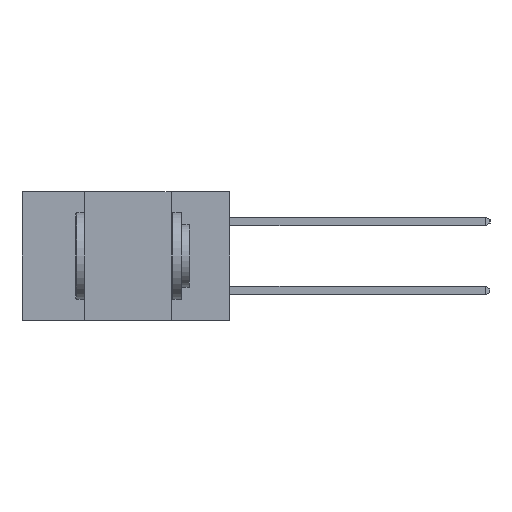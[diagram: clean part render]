
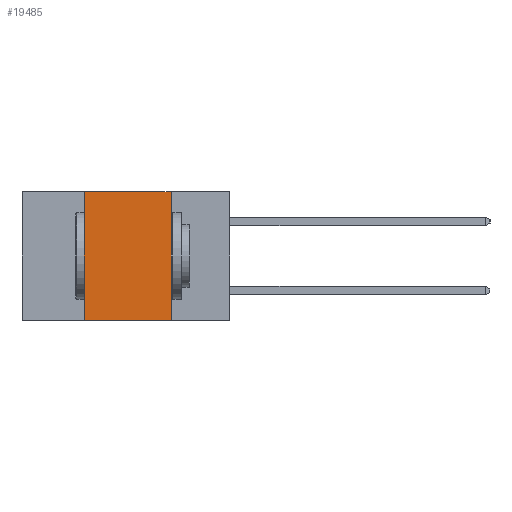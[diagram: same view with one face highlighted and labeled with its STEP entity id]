
A CAD part, left-side view. The second image highlights one B-rep face of the part: STEP entity #19485.
In plain terms, the highlighted planar face has unit normal (-1, 0, 0).
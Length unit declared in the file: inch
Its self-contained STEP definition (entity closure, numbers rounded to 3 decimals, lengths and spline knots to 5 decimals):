
#750 = VERTEX_POINT ( 'NONE', #3642 ) ;
#1356 = VERTEX_POINT ( 'NONE', #4897 ) ;
#1529 = CARTESIAN_POINT ( 'NONE',  ( 0., 0.6, 0. ) ) ;
#2020 = CARTESIAN_POINT ( 'NONE',  ( 0., 0.42, 0. ) ) ;
#2069 = VECTOR ( 'NONE', #5212, 39.37008 ) ;
#2528 = VERTEX_POINT ( 'NONE', #9007 ) ;
#2676 = LINE ( 'NONE', #12717, #2069 ) ;
#3438 = DIRECTION ( 'NONE',  ( 0., -1., 0. ) ) ;
#3642 = CARTESIAN_POINT ( 'NONE',  ( 0., 0.17, 0. ) ) ;
#4897 = CARTESIAN_POINT ( 'NONE',  ( 0., 0.17, -0.37 ) ) ;
#5212 = DIRECTION ( 'NONE',  ( 0., 0., -1. ) ) ;
#6405 = EDGE_CURVE ( 'NONE', #750, #1356, #2676, .T. ) ;
#6628 = LINE ( 'NONE', #1529, #21342 ) ;
#6845 = CARTESIAN_POINT ( 'NONE',  ( 0., 0.42, 0. ) ) ;
#7524 = ORIENTED_EDGE ( 'NONE', *, *, #11236, .F. ) ;
#7940 = LINE ( 'NONE', #8781, #17206 ) ;
#8139 = DIRECTION ( 'NONE',  ( 1., 0., 0. ) ) ;
#8781 = CARTESIAN_POINT ( 'NONE',  ( 0., 0.6, -0.37 ) ) ;
#9007 = CARTESIAN_POINT ( 'NONE',  ( 0., 0.42, -0.37 ) ) ;
#10722 = DIRECTION ( 'NONE',  ( 0., -1., 0. ) ) ;
#11236 = EDGE_CURVE ( 'NONE', #12342, #750, #6628, .T. ) ;
#11530 = FACE_OUTER_BOUND ( 'NONE', #17125, .T. ) ;
#11782 = PLANE ( 'NONE',  #20498 ) ;
#12342 = VERTEX_POINT ( 'NONE', #6845 ) ;
#12434 = ORIENTED_EDGE ( 'NONE', *, *, #22335, .F. ) ;
#12717 = CARTESIAN_POINT ( 'NONE',  ( 0., 0.17, 0. ) ) ;
#15096 = DIRECTION ( 'NONE',  ( 0., 0., 1. ) ) ;
#16526 = VECTOR ( 'NONE', #15096, 39.37008 ) ;
#17125 = EDGE_LOOP ( 'NONE', ( #21072, #7524, #12434, #22789 ) ) ;
#17206 = VECTOR ( 'NONE', #10722, 39.37008 ) ;
#17366 = LINE ( 'NONE', #2020, #16526 ) ;
#19191 = CARTESIAN_POINT ( 'NONE',  ( 0., 0.6, 0. ) ) ;
#19485 = ADVANCED_FACE ( 'NONE', ( #11530 ), #11782, .F. ) ;
#20498 = AXIS2_PLACEMENT_3D ( 'NONE', #19191, #8139, #21042 ) ;
#21042 = DIRECTION ( 'NONE',  ( 0., 0., -1. ) ) ;
#21072 = ORIENTED_EDGE ( 'NONE', *, *, #6405, .F. ) ;
#21342 = VECTOR ( 'NONE', #3438, 39.37008 ) ;
#21704 = EDGE_CURVE ( 'NONE', #2528, #1356, #7940, .T. ) ;
#22335 = EDGE_CURVE ( 'NONE', #2528, #12342, #17366, .T. ) ;
#22789 = ORIENTED_EDGE ( 'NONE', *, *, #21704, .T. ) ;
